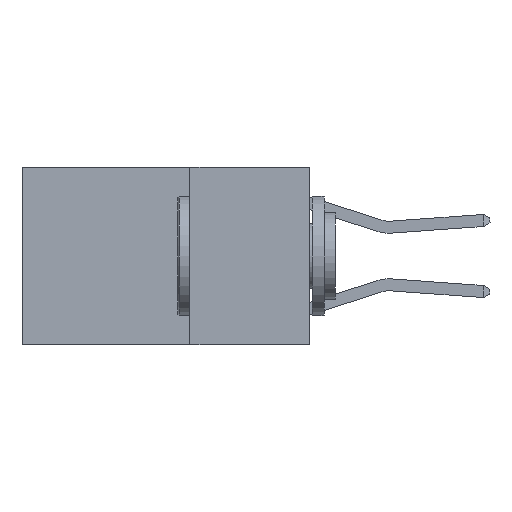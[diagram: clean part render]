
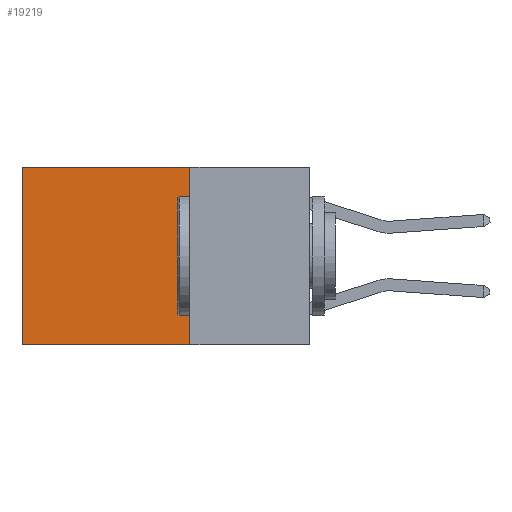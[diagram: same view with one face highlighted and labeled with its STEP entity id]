
A CAD part, left-side view. The second image highlights one B-rep face of the part: STEP entity #19219.
In plain terms, the highlighted planar face has unit normal (-1, 0, 0).
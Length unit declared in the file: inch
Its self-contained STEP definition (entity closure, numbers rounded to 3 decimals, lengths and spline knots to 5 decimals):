
#25 = DIRECTION ( 'NONE',  ( 0., 1., 0. ) ) ;
#1263 = LINE ( 'NONE', #18575, #17113 ) ;
#1297 = DIRECTION ( 'NONE',  ( 0., 1., 0. ) ) ;
#2533 = LINE ( 'NONE', #10211, #6124 ) ;
#2871 = EDGE_CURVE ( 'NONE', #8021, #18009, #7370, .T. ) ;
#2893 = VERTEX_POINT ( 'NONE', #12341 ) ;
#3045 = CARTESIAN_POINT ( 'NONE',  ( 0.2625, 0.25, 0. ) ) ;
#3148 = DIRECTION ( 'NONE',  ( 0., 0., -1. ) ) ;
#4440 = FACE_OUTER_BOUND ( 'NONE', #17863, .T. ) ;
#5152 = PLANE ( 'NONE',  #12682 ) ;
#5405 = CARTESIAN_POINT ( 'NONE',  ( 0.2625, 0.25, -0.37 ) ) ;
#6124 = VECTOR ( 'NONE', #11758, 39.37008 ) ;
#6700 = DIRECTION ( 'NONE',  ( 1., 0., 0. ) ) ;
#7370 = LINE ( 'NONE', #3045, #10984 ) ;
#7628 = EDGE_CURVE ( 'NONE', #8021, #19371, #1263, .T. ) ;
#8021 = VERTEX_POINT ( 'NONE', #14927 ) ;
#9453 = ORIENTED_EDGE ( 'NONE', *, *, #2871, .T. ) ;
#9518 = ORIENTED_EDGE ( 'NONE', *, *, #14620, .T. ) ;
#10211 = CARTESIAN_POINT ( 'NONE',  ( 0.2625, 0.6, 0. ) ) ;
#10984 = VECTOR ( 'NONE', #25, 39.37008 ) ;
#11758 = DIRECTION ( 'NONE',  ( 0., 0., -1. ) ) ;
#12011 = CARTESIAN_POINT ( 'NONE',  ( 0.2625, 0.25, -0.37 ) ) ;
#12341 = CARTESIAN_POINT ( 'NONE',  ( 0.2625, 0.6, -0.37 ) ) ;
#12682 = AXIS2_PLACEMENT_3D ( 'NONE', #18964, #6700, #17486 ) ;
#12871 = VECTOR ( 'NONE', #1297, 39.37008 ) ;
#14620 = EDGE_CURVE ( 'NONE', #18009, #2893, #2533, .T. ) ;
#14688 = CARTESIAN_POINT ( 'NONE',  ( 0.2625, 0.6, 0. ) ) ;
#14927 = CARTESIAN_POINT ( 'NONE',  ( 0.2625, 0.25, 0. ) ) ;
#16193 = ORIENTED_EDGE ( 'NONE', *, *, #7628, .F. ) ;
#16980 = LINE ( 'NONE', #12011, #12871 ) ;
#17113 = VECTOR ( 'NONE', #3148, 39.37008 ) ;
#17486 = DIRECTION ( 'NONE',  ( 0., 0., -1. ) ) ;
#17683 = ORIENTED_EDGE ( 'NONE', *, *, #19443, .F. ) ;
#17863 = EDGE_LOOP ( 'NONE', ( #9518, #17683, #16193, #9453 ) ) ;
#18009 = VERTEX_POINT ( 'NONE', #14688 ) ;
#18575 = CARTESIAN_POINT ( 'NONE',  ( 0.2625, 0.25, 0. ) ) ;
#18964 = CARTESIAN_POINT ( 'NONE',  ( 0.2625, 0.25, 0. ) ) ;
#19219 = ADVANCED_FACE ( 'NONE', ( #4440 ), #5152, .F. ) ;
#19371 = VERTEX_POINT ( 'NONE', #5405 ) ;
#19443 = EDGE_CURVE ( 'NONE', #19371, #2893, #16980, .T. ) ;
